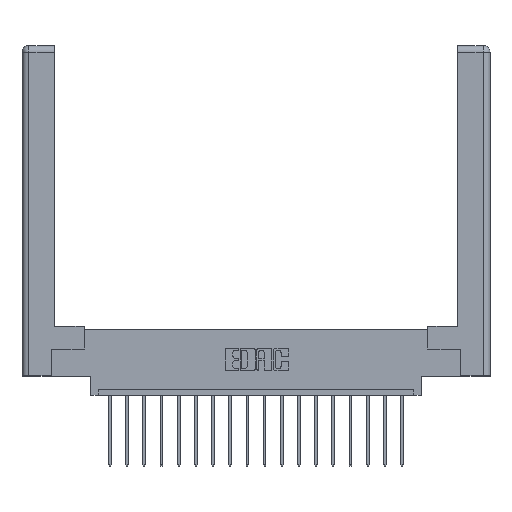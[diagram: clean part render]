
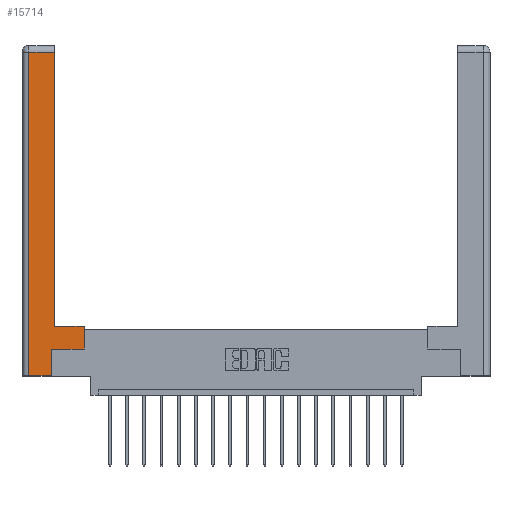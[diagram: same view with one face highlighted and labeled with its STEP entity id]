
A CAD part, top view. The second image highlights one B-rep face of the part: STEP entity #15714.
In plain terms, the highlighted planar face has unit normal (0, 0, 1).
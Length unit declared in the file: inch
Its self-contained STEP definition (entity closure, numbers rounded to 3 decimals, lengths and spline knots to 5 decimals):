
#102 = VERTEX_POINT ( 'NONE', #1162 ) ;
#250 = VECTOR ( 'NONE', #5471, 39.37008 ) ;
#376 = CARTESIAN_POINT ( 'NONE',  ( 0.565, 0.245, 0. ) ) ;
#377 = VERTEX_POINT ( 'NONE', #583 ) ;
#504 = EDGE_CURVE ( 'NONE', #8199, #7188, #15150, .T. ) ;
#583 = CARTESIAN_POINT ( 'NONE',  ( 0.565, 0.245, 0. ) ) ;
#806 = VERTEX_POINT ( 'NONE', #4414 ) ;
#915 = DIRECTION ( 'NONE',  ( -1., 0., 0. ) ) ;
#1162 = CARTESIAN_POINT ( 'NONE',  ( 0.295, 0.45, 0. ) ) ;
#1728 = ORIENTED_EDGE ( 'NONE', *, *, #15433, .T. ) ;
#2110 = CARTESIAN_POINT ( 'NONE',  ( 0.295, 0.45, 0. ) ) ;
#2269 = AXIS2_PLACEMENT_3D ( 'NONE', #7232, #14520, #8802 ) ;
#2625 = DIRECTION ( 'NONE',  ( 1., 0., 0. ) ) ;
#2912 = PLANE ( 'NONE',  #2269 ) ;
#3089 = LINE ( 'NONE', #376, #17965 ) ;
#4414 = CARTESIAN_POINT ( 'NONE',  ( 0.265, 0., 0. ) ) ;
#4453 = DIRECTION ( 'NONE',  ( 0., 1., 0. ) ) ;
#4475 = FACE_OUTER_BOUND ( 'NONE', #13968, .T. ) ;
#4525 = CARTESIAN_POINT ( 'NONE',  ( 0.565, 0.45, 0. ) ) ;
#5234 = EDGE_CURVE ( 'NONE', #14607, #377, #3089, .T. ) ;
#5471 = DIRECTION ( 'NONE',  ( 0., -1., 0. ) ) ;
#5831 = CARTESIAN_POINT ( 'NONE',  ( 0.295, 2.94, 0. ) ) ;
#5952 = EDGE_CURVE ( 'NONE', #13892, #8199, #15181, .T. ) ;
#6193 = DIRECTION ( 'NONE',  ( 0., 1., 0. ) ) ;
#6633 = ORIENTED_EDGE ( 'NONE', *, *, #13890, .T. ) ;
#6976 = LINE ( 'NONE', #18903, #7686 ) ;
#7188 = VERTEX_POINT ( 'NONE', #13361 ) ;
#7232 = CARTESIAN_POINT ( 'NONE',  ( 0., 0., 0. ) ) ;
#7446 = ORIENTED_EDGE ( 'NONE', *, *, #5952, .T. ) ;
#7567 = VECTOR ( 'NONE', #13467, 39.37008 ) ;
#7686 = VECTOR ( 'NONE', #2625, 39.37008 ) ;
#8171 = LINE ( 'NONE', #15324, #18418 ) ;
#8199 = VERTEX_POINT ( 'NONE', #17794 ) ;
#8447 = CARTESIAN_POINT ( 'NONE',  ( 0.0615, 0., 0. ) ) ;
#8802 = DIRECTION ( 'NONE',  ( -1., 0., 0. ) ) ;
#9251 = CARTESIAN_POINT ( 'NONE',  ( 0.295, 3., 0. ) ) ;
#10865 = VERTEX_POINT ( 'NONE', #11296 ) ;
#10911 = EDGE_CURVE ( 'NONE', #7188, #806, #6976, .T. ) ;
#10964 = VECTOR ( 'NONE', #915, 39.37008 ) ;
#11296 = CARTESIAN_POINT ( 'NONE',  ( 0.565, 0.45, 0. ) ) ;
#11516 = ORIENTED_EDGE ( 'NONE', *, *, #10911, .T. ) ;
#11577 = ORIENTED_EDGE ( 'NONE', *, *, #16642, .T. ) ;
#11975 = LINE ( 'NONE', #9251, #7567 ) ;
#13094 = LINE ( 'NONE', #2110, #18202 ) ;
#13361 = CARTESIAN_POINT ( 'NONE',  ( 0.0615, 0., 0. ) ) ;
#13467 = DIRECTION ( 'NONE',  ( 0., 1., 0. ) ) ;
#13890 = EDGE_CURVE ( 'NONE', #377, #10865, #18948, .T. ) ;
#13892 = VERTEX_POINT ( 'NONE', #5831 ) ;
#13968 = EDGE_LOOP ( 'NONE', ( #11577, #7446, #16743, #11516, #17434, #17988, #6633, #1728 ) ) ;
#14132 = DIRECTION ( 'NONE',  ( -1., 0., 0. ) ) ;
#14520 = DIRECTION ( 'NONE',  ( 0., 0., -1. ) ) ;
#14607 = VERTEX_POINT ( 'NONE', #19033 ) ;
#15150 = LINE ( 'NONE', #8447, #250 ) ;
#15181 = LINE ( 'NONE', #16778, #10964 ) ;
#15324 = CARTESIAN_POINT ( 'NONE',  ( 0.265, 0.245, 0. ) ) ;
#15433 = EDGE_CURVE ( 'NONE', #10865, #102, #13094, .T. ) ;
#15714 = ADVANCED_FACE ( 'NONE', ( #4475 ), #2912, .F. ) ;
#16642 = EDGE_CURVE ( 'NONE', #102, #13892, #11975, .T. ) ;
#16743 = ORIENTED_EDGE ( 'NONE', *, *, #504, .T. ) ;
#16778 = CARTESIAN_POINT ( 'NONE',  ( 0.0615, 2.94, 0. ) ) ;
#17169 = DIRECTION ( 'NONE',  ( 1., 0., 0. ) ) ;
#17434 = ORIENTED_EDGE ( 'NONE', *, *, #18454, .T. ) ;
#17794 = CARTESIAN_POINT ( 'NONE',  ( 0.0615, 2.94, 0. ) ) ;
#17965 = VECTOR ( 'NONE', #17169, 39.37008 ) ;
#17988 = ORIENTED_EDGE ( 'NONE', *, *, #5234, .T. ) ;
#18202 = VECTOR ( 'NONE', #14132, 39.37008 ) ;
#18418 = VECTOR ( 'NONE', #6193, 39.37008 ) ;
#18454 = EDGE_CURVE ( 'NONE', #806, #14607, #8171, .T. ) ;
#18488 = VECTOR ( 'NONE', #4453, 39.37008 ) ;
#18903 = CARTESIAN_POINT ( 'NONE',  ( 0.265, 0., 0. ) ) ;
#18948 = LINE ( 'NONE', #4525, #18488 ) ;
#19033 = CARTESIAN_POINT ( 'NONE',  ( 0.265, 0.245, 0. ) ) ;
